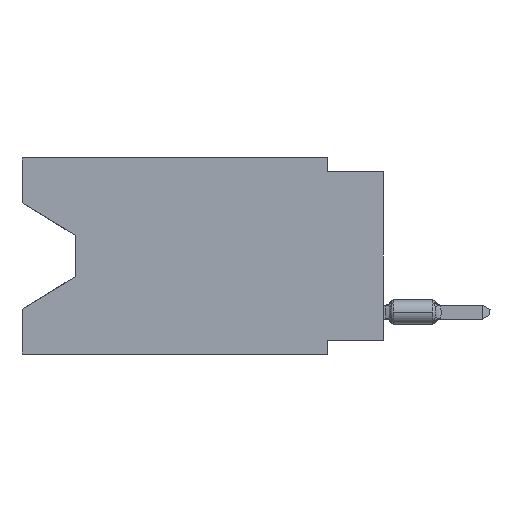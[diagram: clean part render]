
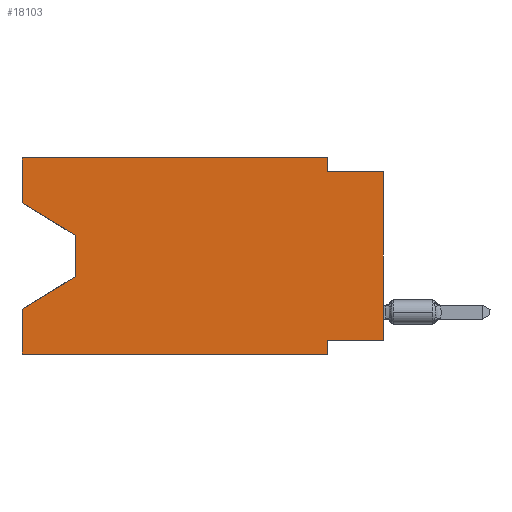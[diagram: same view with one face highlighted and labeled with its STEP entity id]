
A CAD part, left-side view. The second image highlights one B-rep face of the part: STEP entity #18103.
In plain terms, the highlighted planar face has unit normal (-1, 0, 0).
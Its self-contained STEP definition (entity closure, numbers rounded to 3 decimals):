
#558 = LINE ( 'NONE', #19283, #10753 ) ;
#717 = ORIENTED_EDGE ( 'NONE', *, *, #20411, .F. ) ;
#922 = LINE ( 'NONE', #13001, #23248 ) ;
#981 = LINE ( 'NONE', #37999, #15201 ) ;
#1175 = CARTESIAN_POINT ( 'NONE',  ( 0., 13.97, -3.505 ) ) ;
#1430 = ORIENTED_EDGE ( 'NONE', *, *, #23866, .T. ) ;
#1461 = EDGE_CURVE ( 'NONE', #19670, #36053, #37868, .T. ) ;
#2260 = ORIENTED_EDGE ( 'NONE', *, *, #37238, .F. ) ;
#2928 = CARTESIAN_POINT ( 'NONE',  ( 0., 0., -0.635 ) ) ;
#3684 = EDGE_LOOP ( 'NONE', ( #1430, #7433, #28002, #717, #25109, #5571, #2260, #34795, #21357, #32522, #10405, #4334 ) ) ;
#4334 = ORIENTED_EDGE ( 'NONE', *, *, #9775, .F. ) ;
#4611 = DIRECTION ( 'NONE',  ( 0., 0., 1. ) ) ;
#4870 = EDGE_CURVE ( 'NONE', #16953, #36053, #26518, .T. ) ;
#5571 = ORIENTED_EDGE ( 'NONE', *, *, #32504, .F. ) ;
#5606 = CARTESIAN_POINT ( 'NONE',  ( 0., 0., -8.255 ) ) ;
#6095 = VERTEX_POINT ( 'NONE', #15350 ) ;
#6935 = VERTEX_POINT ( 'NONE', #21937 ) ;
#7023 = DIRECTION ( 'NONE',  ( 0., 0.855, -0.519 ) ) ;
#7039 = CARTESIAN_POINT ( 'NONE',  ( 0., 16.383, 0. ) ) ;
#7433 = ORIENTED_EDGE ( 'NONE', *, *, #19481, .T. ) ;
#7518 = CARTESIAN_POINT ( 'NONE',  ( 0., 2.54, -8.89 ) ) ;
#7522 = VERTEX_POINT ( 'NONE', #18564 ) ;
#7748 = VECTOR ( 'NONE', #22314, 1000. ) ;
#8171 = PLANE ( 'NONE',  #16659 ) ;
#8177 = CARTESIAN_POINT ( 'NONE',  ( 0., 13.97, -3.505 ) ) ;
#8777 = DIRECTION ( 'NONE',  ( 1., 0., 0. ) ) ;
#9593 = VERTEX_POINT ( 'NONE', #7039 ) ;
#9775 = EDGE_CURVE ( 'NONE', #23696, #9593, #24196, .T. ) ;
#10307 = DIRECTION ( 'NONE',  ( 0., -1., 0. ) ) ;
#10405 = ORIENTED_EDGE ( 'NONE', *, *, #38164, .F. ) ;
#10753 = VECTOR ( 'NONE', #34962, 1000. ) ;
#11075 = EDGE_CURVE ( 'NONE', #6935, #24229, #22772, .T. ) ;
#11128 = CARTESIAN_POINT ( 'NONE',  ( 0., 2.54, 0. ) ) ;
#12182 = DIRECTION ( 'NONE',  ( 0., 0., 1. ) ) ;
#12787 = LINE ( 'NONE', #16211, #19952 ) ;
#12829 = VECTOR ( 'NONE', #20454, 1000. ) ;
#13001 = CARTESIAN_POINT ( 'NONE',  ( 0., 16.383, -2.038 ) ) ;
#13215 = EDGE_CURVE ( 'NONE', #37746, #6095, #981, .T. ) ;
#14672 = VERTEX_POINT ( 'NONE', #24282 ) ;
#15201 = VECTOR ( 'NONE', #7023, 1000. ) ;
#15350 = CARTESIAN_POINT ( 'NONE',  ( 0., 16.383, -6.852 ) ) ;
#15372 = LINE ( 'NONE', #36889, #26985 ) ;
#15833 = CARTESIAN_POINT ( 'NONE',  ( 0., 16.383, -2.038 ) ) ;
#16211 = CARTESIAN_POINT ( 'NONE',  ( 0., 16.383, 0. ) ) ;
#16659 = AXIS2_PLACEMENT_3D ( 'NONE', #30117, #8777, #26481 ) ;
#16953 = VERTEX_POINT ( 'NONE', #5606 ) ;
#17449 = DIRECTION ( 'NONE',  ( 0., 1., 0. ) ) ;
#18103 = ADVANCED_FACE ( 'NONE', ( #32150 ), #8171, .F. ) ;
#18564 = CARTESIAN_POINT ( 'NONE',  ( 0., 2.54, -8.255 ) ) ;
#18882 = VECTOR ( 'NONE', #36066, 1000. ) ;
#19283 = CARTESIAN_POINT ( 'NONE',  ( 0., 2.54, -8.89 ) ) ;
#19298 = CARTESIAN_POINT ( 'NONE',  ( 0., 16.383, 0. ) ) ;
#19481 = EDGE_CURVE ( 'NONE', #38289, #37746, #26884, .T. ) ;
#19670 = VERTEX_POINT ( 'NONE', #35109 ) ;
#19951 = DIRECTION ( 'NONE',  ( 0., -1., 0. ) ) ;
#19952 = VECTOR ( 'NONE', #12182, 1000. ) ;
#20411 = EDGE_CURVE ( 'NONE', #6935, #6095, #12787, .T. ) ;
#20454 = DIRECTION ( 'NONE',  ( 0., 0., -1. ) ) ;
#21357 = ORIENTED_EDGE ( 'NONE', *, *, #1461, .F. ) ;
#21937 = CARTESIAN_POINT ( 'NONE',  ( 0., 16.383, -8.89 ) ) ;
#22314 = DIRECTION ( 'NONE',  ( 0., -1., 0. ) ) ;
#22772 = LINE ( 'NONE', #35034, #28485 ) ;
#23248 = VECTOR ( 'NONE', #34722, 1000. ) ;
#23606 = LINE ( 'NONE', #11128, #18882 ) ;
#23696 = VERTEX_POINT ( 'NONE', #15833 ) ;
#23866 = EDGE_CURVE ( 'NONE', #23696, #38289, #922, .T. ) ;
#24196 = LINE ( 'NONE', #33636, #34804 ) ;
#24229 = VERTEX_POINT ( 'NONE', #7518 ) ;
#24282 = CARTESIAN_POINT ( 'NONE',  ( 0., 2.54, 0. ) ) ;
#25109 = ORIENTED_EDGE ( 'NONE', *, *, #11075, .T. ) ;
#25567 = VECTOR ( 'NONE', #4611, 1000. ) ;
#26333 = CARTESIAN_POINT ( 'NONE',  ( 0., 0., 0. ) ) ;
#26481 = DIRECTION ( 'NONE',  ( 0., 0., -1. ) ) ;
#26518 = LINE ( 'NONE', #26333, #25567 ) ;
#26884 = LINE ( 'NONE', #8177, #12829 ) ;
#26985 = VECTOR ( 'NONE', #17449, 1000. ) ;
#27910 = EDGE_CURVE ( 'NONE', #14672, #19670, #23606, .T. ) ;
#27997 = CARTESIAN_POINT ( 'NONE',  ( 0., 13.97, -5.385 ) ) ;
#28002 = ORIENTED_EDGE ( 'NONE', *, *, #13215, .T. ) ;
#28354 = LINE ( 'NONE', #19298, #7748 ) ;
#28485 = VECTOR ( 'NONE', #19951, 1000. ) ;
#30117 = CARTESIAN_POINT ( 'NONE',  ( 0., 16.383, 0. ) ) ;
#30448 = DIRECTION ( 'NONE',  ( 0., 0., 1. ) ) ;
#32150 = FACE_OUTER_BOUND ( 'NONE', #3684, .T. ) ;
#32504 = EDGE_CURVE ( 'NONE', #7522, #24229, #558, .T. ) ;
#32522 = ORIENTED_EDGE ( 'NONE', *, *, #27910, .F. ) ;
#33636 = CARTESIAN_POINT ( 'NONE',  ( 0., 16.383, 0. ) ) ;
#34722 = DIRECTION ( 'NONE',  ( 0., -0.855, -0.519 ) ) ;
#34795 = ORIENTED_EDGE ( 'NONE', *, *, #4870, .T. ) ;
#34804 = VECTOR ( 'NONE', #30448, 1000. ) ;
#34962 = DIRECTION ( 'NONE',  ( 0., 0., -1. ) ) ;
#35034 = CARTESIAN_POINT ( 'NONE',  ( 0., 16.383, -8.89 ) ) ;
#35109 = CARTESIAN_POINT ( 'NONE',  ( 0., 2.54, -0.635 ) ) ;
#36053 = VERTEX_POINT ( 'NONE', #37229 ) ;
#36066 = DIRECTION ( 'NONE',  ( 0., 0., -1. ) ) ;
#36226 = VECTOR ( 'NONE', #10307, 1000. ) ;
#36889 = CARTESIAN_POINT ( 'NONE',  ( 0., 0., -8.255 ) ) ;
#37229 = CARTESIAN_POINT ( 'NONE',  ( 0., 0., -0.635 ) ) ;
#37238 = EDGE_CURVE ( 'NONE', #16953, #7522, #15372, .T. ) ;
#37746 = VERTEX_POINT ( 'NONE', #27997 ) ;
#37868 = LINE ( 'NONE', #2928, #36226 ) ;
#37999 = CARTESIAN_POINT ( 'NONE',  ( 0., 13.97, -5.385 ) ) ;
#38164 = EDGE_CURVE ( 'NONE', #9593, #14672, #28354, .T. ) ;
#38289 = VERTEX_POINT ( 'NONE', #1175 ) ;
